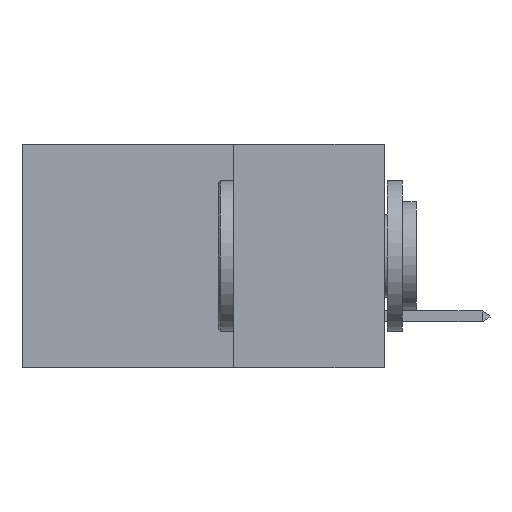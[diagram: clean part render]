
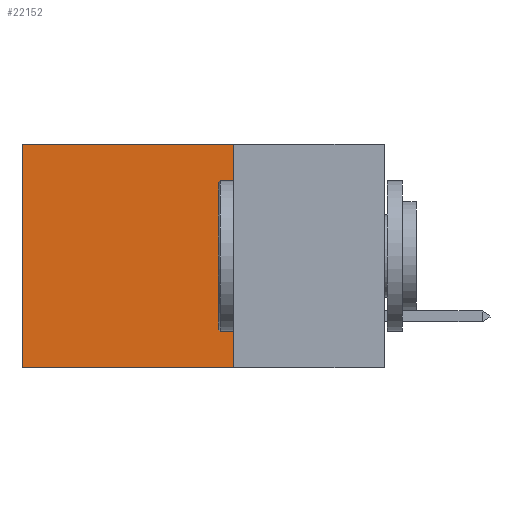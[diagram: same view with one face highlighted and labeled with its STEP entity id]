
A CAD part, left-side view. The second image highlights one B-rep face of the part: STEP entity #22152.
In plain terms, the highlighted planar face has unit normal (-1, 0, 0).
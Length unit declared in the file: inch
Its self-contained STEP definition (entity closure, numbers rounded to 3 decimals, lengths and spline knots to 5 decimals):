
#1099 = PLANE ( 'NONE',  #12583 ) ;
#1347 = EDGE_CURVE ( 'NONE', #13697, #7427, #17830, .T. ) ;
#1891 = VERTEX_POINT ( 'NONE', #20954 ) ;
#3081 = EDGE_CURVE ( 'NONE', #19327, #13697, #23438, .T. ) ;
#3124 = CARTESIAN_POINT ( 'NONE',  ( 0.2875, 0.25, 0. ) ) ;
#3513 = ORIENTED_EDGE ( 'NONE', *, *, #3081, .T. ) ;
#5009 = ORIENTED_EDGE ( 'NONE', *, *, #22159, .F. ) ;
#5190 = DIRECTION ( 'NONE',  ( 0., 0., -1. ) ) ;
#5336 = CARTESIAN_POINT ( 'NONE',  ( 0.2875, 0.6, 0. ) ) ;
#7230 = CARTESIAN_POINT ( 'NONE',  ( 0.2875, 0.25, 0. ) ) ;
#7257 = VECTOR ( 'NONE', #20788, 39.37008 ) ;
#7427 = VERTEX_POINT ( 'NONE', #16512 ) ;
#10222 = DIRECTION ( 'NONE',  ( 0., 1., 0. ) ) ;
#10986 = CARTESIAN_POINT ( 'NONE',  ( 0.2875, 0.6, 0. ) ) ;
#11921 = EDGE_LOOP ( 'NONE', ( #19844, #18280, #5009, #3513 ) ) ;
#12583 = AXIS2_PLACEMENT_3D ( 'NONE', #3124, #17163, #5190 ) ;
#12967 = VECTOR ( 'NONE', #19308, 39.37008 ) ;
#13697 = VERTEX_POINT ( 'NONE', #10986 ) ;
#13751 = VECTOR ( 'NONE', #10222, 39.37008 ) ;
#14541 = FACE_OUTER_BOUND ( 'NONE', #11921, .T. ) ;
#16512 = CARTESIAN_POINT ( 'NONE',  ( 0.2875, 0.6, -0.37 ) ) ;
#17163 = DIRECTION ( 'NONE',  ( 1., 0., 0. ) ) ;
#17379 = CARTESIAN_POINT ( 'NONE',  ( 0.2875, 0.25, -0.37 ) ) ;
#17830 = LINE ( 'NONE', #5336, #7257 ) ;
#17936 = CARTESIAN_POINT ( 'NONE',  ( 0.2875, 0.25, 0. ) ) ;
#18280 = ORIENTED_EDGE ( 'NONE', *, *, #22828, .F. ) ;
#18789 = LINE ( 'NONE', #17379, #12967 ) ;
#19099 = DIRECTION ( 'NONE',  ( 0., 0., -1. ) ) ;
#19308 = DIRECTION ( 'NONE',  ( 0., 1., 0. ) ) ;
#19327 = VERTEX_POINT ( 'NONE', #17936 ) ;
#19713 = LINE ( 'NONE', #7230, #24815 ) ;
#19844 = ORIENTED_EDGE ( 'NONE', *, *, #1347, .T. ) ;
#20788 = DIRECTION ( 'NONE',  ( 0., 0., -1. ) ) ;
#20954 = CARTESIAN_POINT ( 'NONE',  ( 0.2875, 0.25, -0.37 ) ) ;
#21908 = CARTESIAN_POINT ( 'NONE',  ( 0.2875, 0.25, 0. ) ) ;
#22152 = ADVANCED_FACE ( 'NONE', ( #14541 ), #1099, .F. ) ;
#22159 = EDGE_CURVE ( 'NONE', #19327, #1891, #19713, .T. ) ;
#22828 = EDGE_CURVE ( 'NONE', #1891, #7427, #18789, .T. ) ;
#23438 = LINE ( 'NONE', #21908, #13751 ) ;
#24815 = VECTOR ( 'NONE', #19099, 39.37008 ) ;
